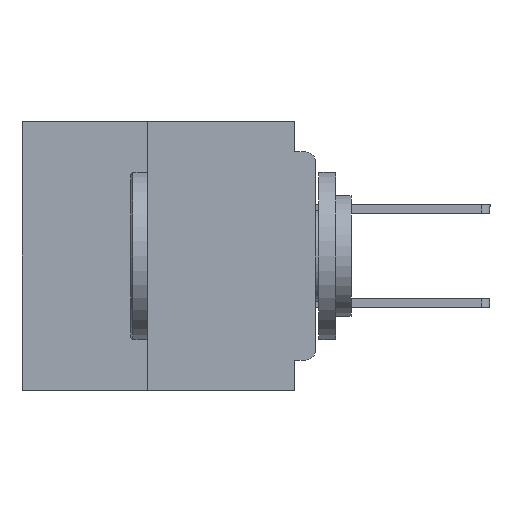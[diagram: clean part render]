
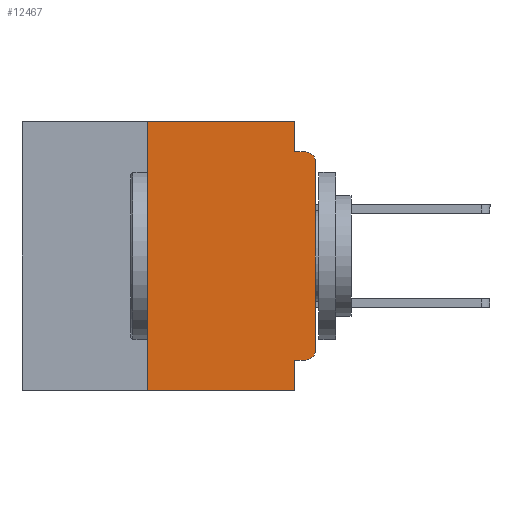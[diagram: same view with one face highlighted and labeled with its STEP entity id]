
A CAD part, left-side view. The second image highlights one B-rep face of the part: STEP entity #12467.
In plain terms, the highlighted planar face has unit normal (-1, 0, 0).
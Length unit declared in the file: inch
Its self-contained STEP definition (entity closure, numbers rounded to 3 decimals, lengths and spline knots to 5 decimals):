
#52 = LINE ( 'NONE', #41726, #27739 ) ;
#724 = VECTOR ( 'NONE', #30969, 39.37008 ) ;
#1365 = VECTOR ( 'NONE', #27259, 39.37008 ) ;
#1421 = CARTESIAN_POINT ( 'NONE',  ( 0., 0.437, 0. ) ) ;
#1444 = CARTESIAN_POINT ( 'NONE',  ( 0., 0.25, -0.4 ) ) ;
#2292 = CARTESIAN_POINT ( 'NONE',  ( 0., 0., -0.355 ) ) ;
#2363 = EDGE_CURVE ( 'NONE', #45218, #13233, #20662, .T. ) ;
#2532 = VERTEX_POINT ( 'NONE', #18339 ) ;
#5115 = PLANE ( 'NONE',  #26014 ) ;
#5147 = ORIENTED_EDGE ( 'NONE', *, *, #28613, .T. ) ;
#5575 = ORIENTED_EDGE ( 'NONE', *, *, #5945, .F. ) ;
#5945 = EDGE_CURVE ( 'NONE', #11521, #2532, #11389, .T. ) ;
#5990 = DIRECTION ( 'NONE',  ( 0., 1., 0. ) ) ;
#6894 = VECTOR ( 'NONE', #5990, 39.37008 ) ;
#7074 = LINE ( 'NONE', #35037, #23971 ) ;
#8164 = EDGE_CURVE ( 'NONE', #30436, #13868, #20700, .T. ) ;
#8485 = CARTESIAN_POINT ( 'NONE',  ( 0., 0.031, -0.4 ) ) ;
#8810 = DIRECTION ( 'NONE',  ( 1., 0., 0. ) ) ;
#9564 = CARTESIAN_POINT ( 'NONE',  ( 0., 0.015, -0.06 ) ) ;
#10011 = VERTEX_POINT ( 'NONE', #37135 ) ;
#10132 = DIRECTION ( 'NONE',  ( 0., -1., 0. ) ) ;
#11133 = VECTOR ( 'NONE', #37129, 39.37008 ) ;
#11347 = CARTESIAN_POINT ( 'NONE',  ( 0., 0.015, -0.34 ) ) ;
#11389 = LINE ( 'NONE', #15641, #18709 ) ;
#11521 = VERTEX_POINT ( 'NONE', #28825 ) ;
#11870 = CIRCLE ( 'NONE', #17407, 0.015 ) ;
#12044 = DIRECTION ( 'NONE',  ( 0., 0., -1. ) ) ;
#12467 = ADVANCED_FACE ( 'NONE', ( #38210 ), #5115, .F. ) ;
#13197 = DIRECTION ( 'NONE',  ( 0., 0., -1. ) ) ;
#13233 = VERTEX_POINT ( 'NONE', #41735 ) ;
#13868 = VERTEX_POINT ( 'NONE', #40500 ) ;
#14104 = EDGE_CURVE ( 'NONE', #38539, #30436, #35535, .T. ) ;
#14971 = ORIENTED_EDGE ( 'NONE', *, *, #2363, .F. ) ;
#14972 = DIRECTION ( 'NONE',  ( 0., 0., -1. ) ) ;
#15257 = EDGE_CURVE ( 'NONE', #10011, #33012, #42684, .T. ) ;
#15641 = CARTESIAN_POINT ( 'NONE',  ( 0., 0.031, 0. ) ) ;
#17106 = AXIS2_PLACEMENT_3D ( 'NONE', #9564, #34636, #13197 ) ;
#17407 = AXIS2_PLACEMENT_3D ( 'NONE', #11347, #36370, #14972 ) ;
#18339 = CARTESIAN_POINT ( 'NONE',  ( 0., 0.031, -0.045 ) ) ;
#18709 = VECTOR ( 'NONE', #12044, 39.37008 ) ;
#20382 = DIRECTION ( 'NONE',  ( 0., 0., 1. ) ) ;
#20662 = LINE ( 'NONE', #27668, #1365 ) ;
#20700 = LINE ( 'NONE', #8485, #11133 ) ;
#23020 = CARTESIAN_POINT ( 'NONE',  ( 0., 0.437, 0. ) ) ;
#23971 = VECTOR ( 'NONE', #10132, 39.37008 ) ;
#25207 = ORIENTED_EDGE ( 'NONE', *, *, #41405, .F. ) ;
#25369 = EDGE_LOOP ( 'NONE', ( #26239, #34739, #25207, #5575, #27378, #14971, #25515, #31752, #28752, #5147 ) ) ;
#25515 = ORIENTED_EDGE ( 'NONE', *, *, #32661, .T. ) ;
#26014 = AXIS2_PLACEMENT_3D ( 'NONE', #1421, #8810, #33913 ) ;
#26239 = ORIENTED_EDGE ( 'NONE', *, *, #42794, .T. ) ;
#27259 = DIRECTION ( 'NONE',  ( 0., 0., 1. ) ) ;
#27376 = CARTESIAN_POINT ( 'NONE',  ( 0., 0.437, -0.4 ) ) ;
#27378 = ORIENTED_EDGE ( 'NONE', *, *, #46104, .F. ) ;
#27668 = CARTESIAN_POINT ( 'NONE',  ( 0., 0.25, -0.4 ) ) ;
#27739 = VECTOR ( 'NONE', #20382, 39.37008 ) ;
#28613 = EDGE_CURVE ( 'NONE', #38539, #31140, #11870, .T. ) ;
#28752 = ORIENTED_EDGE ( 'NONE', *, *, #14104, .F. ) ;
#28825 = CARTESIAN_POINT ( 'NONE',  ( 0., 0.031, 0. ) ) ;
#29238 = CARTESIAN_POINT ( 'NONE',  ( 0., 0.015, -0.045 ) ) ;
#30001 = VECTOR ( 'NONE', #44322, 39.37008 ) ;
#30436 = VERTEX_POINT ( 'NONE', #43502 ) ;
#30969 = DIRECTION ( 'NONE',  ( 0., -1., 0. ) ) ;
#31140 = VERTEX_POINT ( 'NONE', #39659 ) ;
#31752 = ORIENTED_EDGE ( 'NONE', *, *, #8164, .F. ) ;
#32661 = EDGE_CURVE ( 'NONE', #45218, #13868, #39000, .T. ) ;
#33012 = VERTEX_POINT ( 'NONE', #29238 ) ;
#33913 = DIRECTION ( 'NONE',  ( 0., 0., -1. ) ) ;
#34636 = DIRECTION ( 'NONE',  ( -1., 0., 0. ) ) ;
#34739 = ORIENTED_EDGE ( 'NONE', *, *, #15257, .T. ) ;
#35037 = CARTESIAN_POINT ( 'NONE',  ( 0., 0., -0.045 ) ) ;
#35535 = LINE ( 'NONE', #2292, #6894 ) ;
#36370 = DIRECTION ( 'NONE',  ( -1., 0., 0. ) ) ;
#37129 = DIRECTION ( 'NONE',  ( 0., 0., -1. ) ) ;
#37135 = CARTESIAN_POINT ( 'NONE',  ( 0., 0., -0.06 ) ) ;
#38210 = FACE_OUTER_BOUND ( 'NONE', #25369, .T. ) ;
#38539 = VERTEX_POINT ( 'NONE', #44802 ) ;
#39000 = LINE ( 'NONE', #27376, #724 ) ;
#39477 = LINE ( 'NONE', #23020, #30001 ) ;
#39659 = CARTESIAN_POINT ( 'NONE',  ( 0., 0., -0.34 ) ) ;
#40500 = CARTESIAN_POINT ( 'NONE',  ( 0., 0.031, -0.4 ) ) ;
#41405 = EDGE_CURVE ( 'NONE', #2532, #33012, #7074, .T. ) ;
#41726 = CARTESIAN_POINT ( 'NONE',  ( 0., 0., 0. ) ) ;
#41735 = CARTESIAN_POINT ( 'NONE',  ( 0., 0.25, 0. ) ) ;
#42684 = CIRCLE ( 'NONE', #17106, 0.015 ) ;
#42794 = EDGE_CURVE ( 'NONE', #31140, #10011, #52, .T. ) ;
#43502 = CARTESIAN_POINT ( 'NONE',  ( 0., 0.031, -0.355 ) ) ;
#44322 = DIRECTION ( 'NONE',  ( 0., -1., 0. ) ) ;
#44802 = CARTESIAN_POINT ( 'NONE',  ( 0., 0.015, -0.355 ) ) ;
#45218 = VERTEX_POINT ( 'NONE', #1444 ) ;
#46104 = EDGE_CURVE ( 'NONE', #13233, #11521, #39477, .T. ) ;
